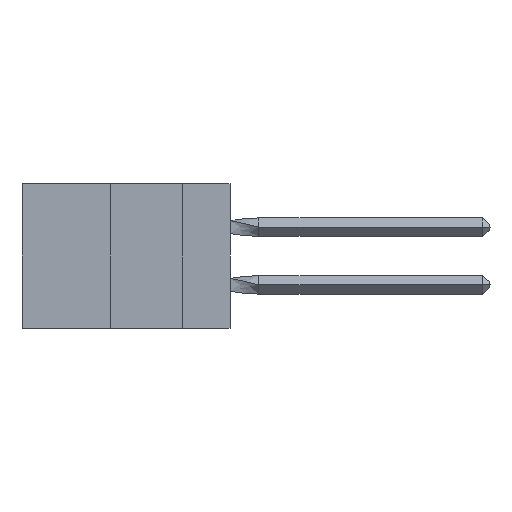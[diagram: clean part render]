
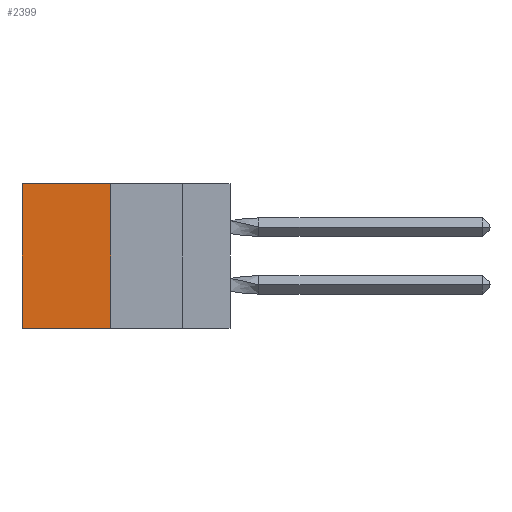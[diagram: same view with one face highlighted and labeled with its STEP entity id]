
A CAD part, left-side view. The second image highlights one B-rep face of the part: STEP entity #2399.
In plain terms, the highlighted planar face has unit normal (-1, 0, 0).
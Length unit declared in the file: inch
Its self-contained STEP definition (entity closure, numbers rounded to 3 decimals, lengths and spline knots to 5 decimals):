
#77 = CARTESIAN_POINT ( 'NONE',  ( 0.305, 0.72, 0. ) ) ;
#224 = ORIENTED_EDGE ( 'NONE', *, *, #13757, .T. ) ;
#762 = EDGE_LOOP ( 'NONE', ( #4310, #3560, #7620, #224 ) ) ;
#1454 = DIRECTION ( 'NONE',  ( 0., 0., -1. ) ) ;
#1868 = VERTEX_POINT ( 'NONE', #14285 ) ;
#2285 = CARTESIAN_POINT ( 'NONE',  ( 0.305, 0.413, -0.5 ) ) ;
#2399 = ADVANCED_FACE ( 'NONE', ( #12619 ), #3151, .F. ) ;
#2636 = EDGE_CURVE ( 'NONE', #15018, #11521, #15997, .T. ) ;
#2762 = DIRECTION ( 'NONE',  ( 0., 1., 0. ) ) ;
#3151 = PLANE ( 'NONE',  #12270 ) ;
#3560 = ORIENTED_EDGE ( 'NONE', *, *, #7611, .F. ) ;
#3818 = DIRECTION ( 'NONE',  ( 0., 0., -1. ) ) ;
#4310 = ORIENTED_EDGE ( 'NONE', *, *, #2636, .T. ) ;
#4471 = DIRECTION ( 'NONE',  ( 0., 0., -1. ) ) ;
#5286 = CARTESIAN_POINT ( 'NONE',  ( 0.305, 0.72, -0.5 ) ) ;
#5417 = VECTOR ( 'NONE', #6273, 39.37008 ) ;
#5810 = LINE ( 'NONE', #8260, #15172 ) ;
#6186 = VECTOR ( 'NONE', #2762, 39.37008 ) ;
#6273 = DIRECTION ( 'NONE',  ( 0., 1., 0. ) ) ;
#7611 = EDGE_CURVE ( 'NONE', #1868, #11521, #14141, .T. ) ;
#7620 = ORIENTED_EDGE ( 'NONE', *, *, #8704, .F. ) ;
#7730 = CARTESIAN_POINT ( 'NONE',  ( 0.305, 0.413, 0. ) ) ;
#8252 = CARTESIAN_POINT ( 'NONE',  ( 0.305, 0.413, 0. ) ) ;
#8260 = CARTESIAN_POINT ( 'NONE',  ( 0.305, 0.413, -0.5 ) ) ;
#8704 = EDGE_CURVE ( 'NONE', #16247, #1868, #5810, .T. ) ;
#10010 = CARTESIAN_POINT ( 'NONE',  ( 0.305, 0.413, -0.5 ) ) ;
#11521 = VERTEX_POINT ( 'NONE', #5286 ) ;
#12270 = AXIS2_PLACEMENT_3D ( 'NONE', #10010, #12683, #4471 ) ;
#12619 = FACE_OUTER_BOUND ( 'NONE', #762, .T. ) ;
#12683 = DIRECTION ( 'NONE',  ( 1., 0., 0. ) ) ;
#12813 = LINE ( 'NONE', #8252, #6186 ) ;
#13757 = EDGE_CURVE ( 'NONE', #16247, #15018, #12813, .T. ) ;
#14141 = LINE ( 'NONE', #2285, #5417 ) ;
#14285 = CARTESIAN_POINT ( 'NONE',  ( 0.305, 0.413, -0.5 ) ) ;
#15018 = VERTEX_POINT ( 'NONE', #77 ) ;
#15172 = VECTOR ( 'NONE', #1454, 39.37008 ) ;
#15997 = LINE ( 'NONE', #17396, #17479 ) ;
#16247 = VERTEX_POINT ( 'NONE', #7730 ) ;
#17396 = CARTESIAN_POINT ( 'NONE',  ( 0.305, 0.72, -0.5 ) ) ;
#17479 = VECTOR ( 'NONE', #3818, 39.37008 ) ;
